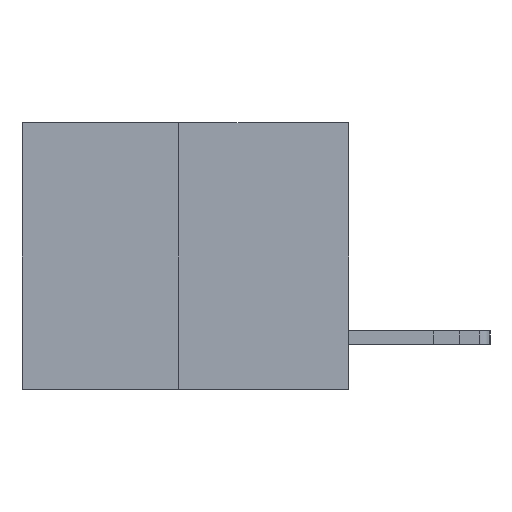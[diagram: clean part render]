
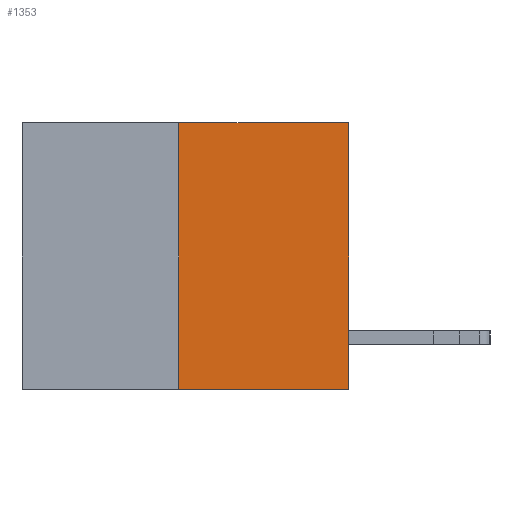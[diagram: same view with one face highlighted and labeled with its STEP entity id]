
A CAD part, left-side view. The second image highlights one B-rep face of the part: STEP entity #1353.
In plain terms, the highlighted planar face has unit normal (-1, 0, 0).
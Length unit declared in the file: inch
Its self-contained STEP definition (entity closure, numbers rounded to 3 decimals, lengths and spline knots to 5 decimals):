
#187 = VECTOR ( 'NONE', #10769, 39.37008 ) ;
#399 = FACE_OUTER_BOUND ( 'NONE', #4586, .T. ) ;
#471 = CARTESIAN_POINT ( 'NONE',  ( 0., 0.6, 0. ) ) ;
#707 = DIRECTION ( 'NONE',  ( 0., 0., -1. ) ) ;
#1053 = LINE ( 'NONE', #471, #10382 ) ;
#1086 = VERTEX_POINT ( 'NONE', #4602 ) ;
#1099 = CARTESIAN_POINT ( 'NONE',  ( 0., 0., -0.49 ) ) ;
#1353 = ADVANCED_FACE ( 'NONE', ( #399 ), #10764, .F. ) ;
#1723 = DIRECTION ( 'NONE',  ( 1., 0., 0. ) ) ;
#2415 = CARTESIAN_POINT ( 'NONE',  ( 0., 0.312, -0.49 ) ) ;
#2816 = CARTESIAN_POINT ( 'NONE',  ( 0., 0., 0. ) ) ;
#2905 = DIRECTION ( 'NONE',  ( 0., 0., 1. ) ) ;
#3254 = CARTESIAN_POINT ( 'NONE',  ( 0., 0.6, -0.49 ) ) ;
#3613 = EDGE_CURVE ( 'NONE', #4051, #1086, #8684, .T. ) ;
#3929 = VECTOR ( 'NONE', #7735, 39.37008 ) ;
#4051 = VERTEX_POINT ( 'NONE', #2415 ) ;
#4586 = EDGE_LOOP ( 'NONE', ( #12529, #12177, #10737, #12924 ) ) ;
#4602 = CARTESIAN_POINT ( 'NONE',  ( 0., 0.312, 0. ) ) ;
#5143 = VECTOR ( 'NONE', #2905, 39.37008 ) ;
#5667 = EDGE_CURVE ( 'NONE', #9714, #8557, #8789, .T. ) ;
#6070 = EDGE_CURVE ( 'NONE', #4051, #9714, #8971, .T. ) ;
#6202 = CARTESIAN_POINT ( 'NONE',  ( 0., 0.6, 0. ) ) ;
#7735 = DIRECTION ( 'NONE',  ( 0., -1., 0. ) ) ;
#8084 = CARTESIAN_POINT ( 'NONE',  ( 0., 0., 0. ) ) ;
#8557 = VERTEX_POINT ( 'NONE', #8084 ) ;
#8684 = LINE ( 'NONE', #11058, #187 ) ;
#8789 = LINE ( 'NONE', #2816, #5143 ) ;
#8971 = LINE ( 'NONE', #3254, #3929 ) ;
#9157 = DIRECTION ( 'NONE',  ( 0., -1., 0. ) ) ;
#9714 = VERTEX_POINT ( 'NONE', #1099 ) ;
#10382 = VECTOR ( 'NONE', #9157, 39.37008 ) ;
#10737 = ORIENTED_EDGE ( 'NONE', *, *, #5667, .T. ) ;
#10764 = PLANE ( 'NONE',  #12851 ) ;
#10769 = DIRECTION ( 'NONE',  ( 0., 0., 1. ) ) ;
#11058 = CARTESIAN_POINT ( 'NONE',  ( 0., 0.312, -0.49 ) ) ;
#12177 = ORIENTED_EDGE ( 'NONE', *, *, #6070, .T. ) ;
#12529 = ORIENTED_EDGE ( 'NONE', *, *, #3613, .F. ) ;
#12851 = AXIS2_PLACEMENT_3D ( 'NONE', #6202, #1723, #707 ) ;
#12924 = ORIENTED_EDGE ( 'NONE', *, *, #13858, .F. ) ;
#13858 = EDGE_CURVE ( 'NONE', #1086, #8557, #1053, .T. ) ;
